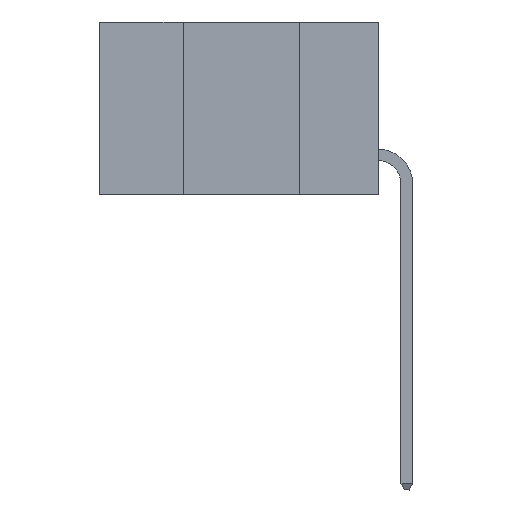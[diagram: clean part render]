
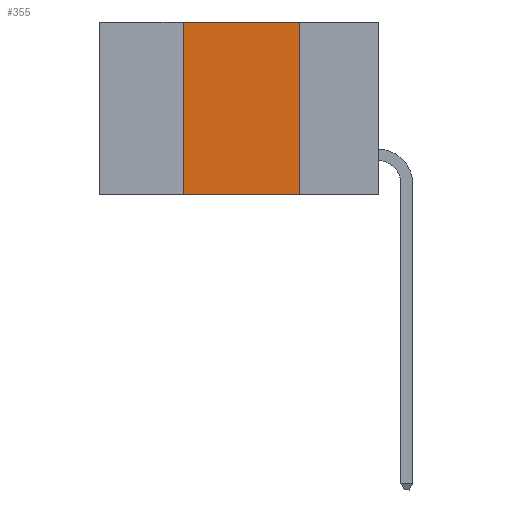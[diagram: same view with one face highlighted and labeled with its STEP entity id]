
A CAD part, left-side view. The second image highlights one B-rep face of the part: STEP entity #355.
In plain terms, the highlighted planar face has unit normal (-1, 0, 0).
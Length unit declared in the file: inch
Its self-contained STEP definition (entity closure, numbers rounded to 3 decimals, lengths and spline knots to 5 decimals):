
#355 = ADVANCED_FACE ( 'NONE', ( #6649 ), #10038, .F. ) ;
#1222 = DIRECTION ( 'NONE',  ( 1., 0., 0. ) ) ;
#1824 = EDGE_CURVE ( 'NONE', #7917, #8535, #9649, .T. ) ;
#2480 = ORIENTED_EDGE ( 'NONE', *, *, #18196, .T. ) ;
#2605 = VERTEX_POINT ( 'NONE', #4568 ) ;
#3260 = CARTESIAN_POINT ( 'NONE',  ( 0., 0.17, -0.37 ) ) ;
#4097 = CARTESIAN_POINT ( 'NONE',  ( 0., 0.6, -0.37 ) ) ;
#4297 = EDGE_CURVE ( 'NONE', #6201, #7917, #9708, .T. ) ;
#4568 = CARTESIAN_POINT ( 'NONE',  ( 0., 0.17, -0.37 ) ) ;
#5651 = ORIENTED_EDGE ( 'NONE', *, *, #10660, .F. ) ;
#5704 = DIRECTION ( 'NONE',  ( 0., -1., 0. ) ) ;
#6201 = VERTEX_POINT ( 'NONE', #15819 ) ;
#6649 = FACE_OUTER_BOUND ( 'NONE', #15794, .T. ) ;
#7164 = VECTOR ( 'NONE', #13733, 39.37008 ) ;
#7917 = VERTEX_POINT ( 'NONE', #18898 ) ;
#8084 = CARTESIAN_POINT ( 'NONE',  ( 0., 0.17, 0. ) ) ;
#8285 = DIRECTION ( 'NONE',  ( 0., 0., -1. ) ) ;
#8535 = VERTEX_POINT ( 'NONE', #8084 ) ;
#9477 = CARTESIAN_POINT ( 'NONE',  ( 0., 0.42, -0.37 ) ) ;
#9649 = LINE ( 'NONE', #18509, #13459 ) ;
#9708 = LINE ( 'NONE', #9477, #13535 ) ;
#10038 = PLANE ( 'NONE',  #21900 ) ;
#10105 = LINE ( 'NONE', #3260, #7164 ) ;
#10660 = EDGE_CURVE ( 'NONE', #8535, #2605, #10105, .T. ) ;
#10854 = VECTOR ( 'NONE', #5704, 39.37008 ) ;
#13459 = VECTOR ( 'NONE', #16783, 39.37008 ) ;
#13535 = VECTOR ( 'NONE', #15098, 39.37008 ) ;
#13733 = DIRECTION ( 'NONE',  ( 0., 0., -1. ) ) ;
#14678 = LINE ( 'NONE', #4097, #10854 ) ;
#15098 = DIRECTION ( 'NONE',  ( 0., 0., 1. ) ) ;
#15794 = EDGE_LOOP ( 'NONE', ( #5651, #20562, #22283, #2480 ) ) ;
#15819 = CARTESIAN_POINT ( 'NONE',  ( 0., 0.42, -0.37 ) ) ;
#16783 = DIRECTION ( 'NONE',  ( 0., -1., 0. ) ) ;
#17156 = CARTESIAN_POINT ( 'NONE',  ( 0., 0.6, 0. ) ) ;
#18196 = EDGE_CURVE ( 'NONE', #6201, #2605, #14678, .T. ) ;
#18509 = CARTESIAN_POINT ( 'NONE',  ( 0., 0.6, 0. ) ) ;
#18898 = CARTESIAN_POINT ( 'NONE',  ( 0., 0.42, 0. ) ) ;
#20562 = ORIENTED_EDGE ( 'NONE', *, *, #1824, .F. ) ;
#21900 = AXIS2_PLACEMENT_3D ( 'NONE', #17156, #1222, #8285 ) ;
#22283 = ORIENTED_EDGE ( 'NONE', *, *, #4297, .F. ) ;
